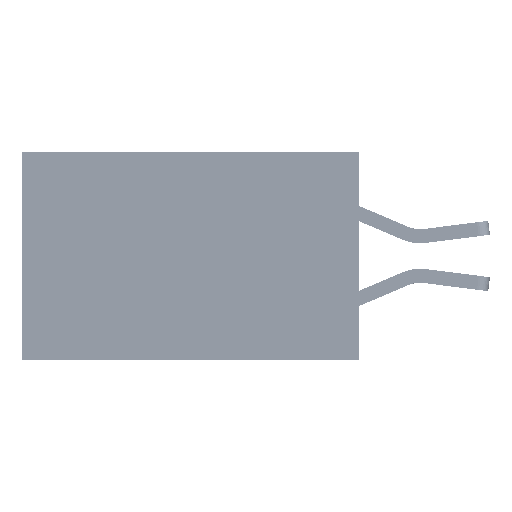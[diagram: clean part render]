
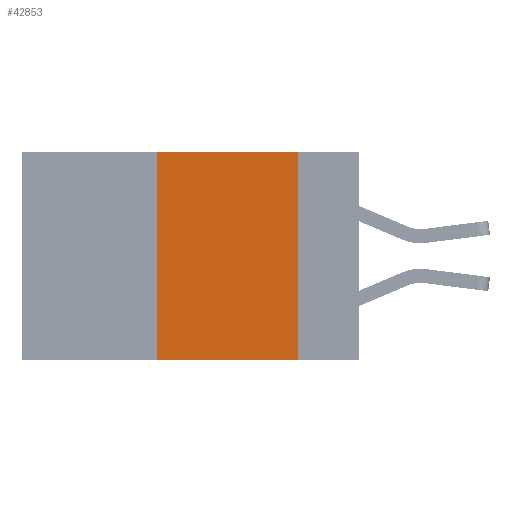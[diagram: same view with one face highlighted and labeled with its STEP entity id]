
A CAD part, left-side view. The second image highlights one B-rep face of the part: STEP entity #42853.
In plain terms, the highlighted planar face has unit normal (-1, 0, 0).
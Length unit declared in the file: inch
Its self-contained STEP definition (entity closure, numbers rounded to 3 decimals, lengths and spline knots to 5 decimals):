
#364 = DIRECTION ( 'NONE',  ( 0., 0., -1. ) ) ;
#2909 = DIRECTION ( 'NONE',  ( 0., 0., -1. ) ) ;
#3236 = DIRECTION ( 'NONE',  ( 0., 0., 1. ) ) ;
#3323 = VERTEX_POINT ( 'NONE', #20007 ) ;
#6177 = ORIENTED_EDGE ( 'NONE', *, *, #11313, .F. ) ;
#6809 = VERTEX_POINT ( 'NONE', #35877 ) ;
#9881 = DIRECTION ( 'NONE',  ( 0., -1., 0. ) ) ;
#10202 = VECTOR ( 'NONE', #11396, 39.37008 ) ;
#11313 = EDGE_CURVE ( 'NONE', #3323, #6809, #45527, .T. ) ;
#11396 = DIRECTION ( 'NONE',  ( 0., -1., 0. ) ) ;
#15896 = VERTEX_POINT ( 'NONE', #31170 ) ;
#17587 = ORIENTED_EDGE ( 'NONE', *, *, #20821, .F. ) ;
#18391 = CARTESIAN_POINT ( 'NONE',  ( 0., 0.6, 0. ) ) ;
#20007 = CARTESIAN_POINT ( 'NONE',  ( 0., 0.36, -0.37 ) ) ;
#20821 = EDGE_CURVE ( 'NONE', #15896, #43692, #42390, .T. ) ;
#20866 = LINE ( 'NONE', #36296, #10202 ) ;
#21954 = DIRECTION ( 'NONE',  ( 1., 0., 0. ) ) ;
#23508 = VECTOR ( 'NONE', #2909, 39.37008 ) ;
#26511 = AXIS2_PLACEMENT_3D ( 'NONE', #18391, #21954, #364 ) ;
#28800 = VECTOR ( 'NONE', #9881, 39.37008 ) ;
#31086 = CARTESIAN_POINT ( 'NONE',  ( 0., 0.6, -0.37 ) ) ;
#31170 = CARTESIAN_POINT ( 'NONE',  ( 0., 0.11, 0. ) ) ;
#31502 = ORIENTED_EDGE ( 'NONE', *, *, #39041, .T. ) ;
#31615 = VECTOR ( 'NONE', #3236, 39.37008 ) ;
#34518 = ORIENTED_EDGE ( 'NONE', *, *, #45778, .F. ) ;
#35877 = CARTESIAN_POINT ( 'NONE',  ( 0., 0.36, 0. ) ) ;
#36296 = CARTESIAN_POINT ( 'NONE',  ( 0., 0.6, 0. ) ) ;
#36485 = EDGE_LOOP ( 'NONE', ( #17587, #34518, #6177, #31502 ) ) ;
#38231 = LINE ( 'NONE', #31086, #28800 ) ;
#38344 = FACE_OUTER_BOUND ( 'NONE', #36485, .T. ) ;
#39041 = EDGE_CURVE ( 'NONE', #3323, #43692, #38231, .T. ) ;
#39558 = CARTESIAN_POINT ( 'NONE',  ( 0., 0.11, -0.37 ) ) ;
#39626 = PLANE ( 'NONE',  #26511 ) ;
#42146 = CARTESIAN_POINT ( 'NONE',  ( 0., 0.11, 0. ) ) ;
#42390 = LINE ( 'NONE', #42146, #23508 ) ;
#42853 = ADVANCED_FACE ( 'NONE', ( #38344 ), #39626, .F. ) ;
#43692 = VERTEX_POINT ( 'NONE', #39558 ) ;
#45527 = LINE ( 'NONE', #46054, #31615 ) ;
#45778 = EDGE_CURVE ( 'NONE', #6809, #15896, #20866, .T. ) ;
#46054 = CARTESIAN_POINT ( 'NONE',  ( 0., 0.36, 0. ) ) ;
